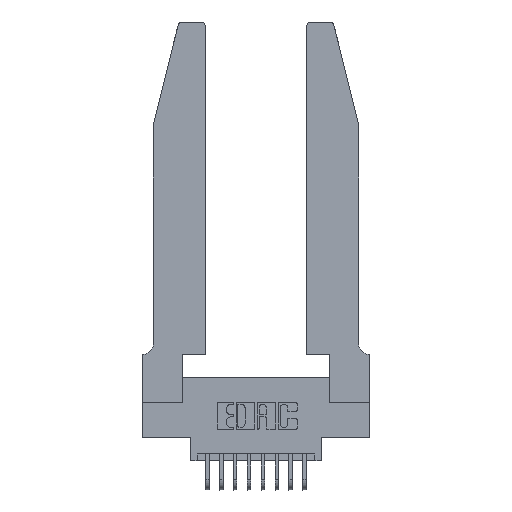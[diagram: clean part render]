
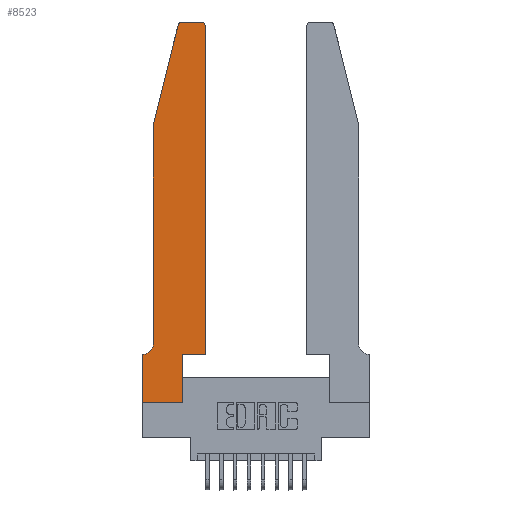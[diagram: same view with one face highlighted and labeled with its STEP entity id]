
A CAD part, top view. The second image highlights one B-rep face of the part: STEP entity #8523.
In plain terms, the highlighted planar face has unit normal (0, 0, 1).
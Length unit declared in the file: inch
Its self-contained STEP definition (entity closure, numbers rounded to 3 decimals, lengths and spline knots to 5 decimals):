
#347 = ORIENTED_EDGE ( 'NONE', *, *, #9754, .T. ) ;
#511 = CARTESIAN_POINT ( 'NONE',  ( 0.2865, 0.35, 0.37 ) ) ;
#692 = VERTEX_POINT ( 'NONE', #4070 ) ;
#704 = EDGE_CURVE ( 'NONE', #1204, #10091, #8605, .T. ) ;
#888 = ORIENTED_EDGE ( 'NONE', *, *, #15218, .T. ) ;
#1204 = VERTEX_POINT ( 'NONE', #12159 ) ;
#1240 = CARTESIAN_POINT ( 'NONE',  ( 0.0755, 2., 0.37 ) ) ;
#1251 = VECTOR ( 'NONE', #17386, 39.37008 ) ;
#1602 = CIRCLE ( 'NONE', #2156, 0.03 ) ;
#1838 = LINE ( 'NONE', #11196, #14035 ) ;
#1917 = DIRECTION ( 'NONE',  ( 1., 0., 0. ) ) ;
#1928 = CARTESIAN_POINT ( 'NONE',  ( 0., 0., 0.37 ) ) ;
#1946 = ORIENTED_EDGE ( 'NONE', *, *, #10575, .T. ) ;
#2156 = AXIS2_PLACEMENT_3D ( 'NONE', #3734, #15535, #12899 ) ;
#2363 = EDGE_CURVE ( 'NONE', #692, #7501, #1602, .T. ) ;
#2417 = CARTESIAN_POINT ( 'NONE',  ( 0.0755, 0.42, 0.37 ) ) ;
#2533 = CARTESIAN_POINT ( 'NONE',  ( 0.2865, 0.35, 0.37 ) ) ;
#2564 = AXIS2_PLACEMENT_3D ( 'NONE', #15201, #5984, #14077 ) ;
#2890 = EDGE_LOOP ( 'NONE', ( #3415, #6520, #11532, #1946, #10622, #15203, #888, #3241, #5533, #347, #11767, #4960 ) ) ;
#3067 = VECTOR ( 'NONE', #17357, 39.37008 ) ;
#3241 = ORIENTED_EDGE ( 'NONE', *, *, #15043, .T. ) ;
#3364 = CARTESIAN_POINT ( 'NONE',  ( 0.4205, 2.72, 0.37 ) ) ;
#3415 = ORIENTED_EDGE ( 'NONE', *, *, #12938, .T. ) ;
#3461 = CARTESIAN_POINT ( 'NONE',  ( 0.4205, 2.75, 0.37 ) ) ;
#3537 = CARTESIAN_POINT ( 'NONE',  ( 0., 0.35, 0.37 ) ) ;
#3642 = VECTOR ( 'NONE', #4032, 39.37008 ) ;
#3734 = CARTESIAN_POINT ( 'NONE',  ( 0.284, 2.72, 0.37 ) ) ;
#4032 = DIRECTION ( 'NONE',  ( 0., -1., 0. ) ) ;
#4070 = CARTESIAN_POINT ( 'NONE',  ( 0.284, 2.75, 0.37 ) ) ;
#4332 = FACE_OUTER_BOUND ( 'NONE', #2890, .T. ) ;
#4350 = AXIS2_PLACEMENT_3D ( 'NONE', #3364, #6073, #15453 ) ;
#4546 = LINE ( 'NONE', #6626, #3067 ) ;
#4590 = VECTOR ( 'NONE', #16129, 39.37008 ) ;
#4960 = ORIENTED_EDGE ( 'NONE', *, *, #11045, .T. ) ;
#4996 = CARTESIAN_POINT ( 'NONE',  ( 0., 0., 0.37 ) ) ;
#5533 = ORIENTED_EDGE ( 'NONE', *, *, #15753, .T. ) ;
#5984 = DIRECTION ( 'NONE',  ( 0., 0., -1. ) ) ;
#6049 = CARTESIAN_POINT ( 'NONE',  ( 0.2865, 0., 0.37 ) ) ;
#6073 = DIRECTION ( 'NONE',  ( 0., 0., 1. ) ) ;
#6252 = DIRECTION ( 'NONE',  ( 1., 0., 0. ) ) ;
#6520 = ORIENTED_EDGE ( 'NONE', *, *, #2363, .T. ) ;
#6537 = CARTESIAN_POINT ( 'NONE',  ( 0.0755, 0.35, 0.37 ) ) ;
#6626 = CARTESIAN_POINT ( 'NONE',  ( 0.4505, 0.35, 0.37 ) ) ;
#6681 = VERTEX_POINT ( 'NONE', #13858 ) ;
#6736 = CARTESIAN_POINT ( 'NONE',  ( 0.0755, 2., 0.37 ) ) ;
#7360 = VERTEX_POINT ( 'NONE', #4996 ) ;
#7501 = VERTEX_POINT ( 'NONE', #15909 ) ;
#7638 = LINE ( 'NONE', #16702, #14593 ) ;
#7845 = EDGE_CURVE ( 'NONE', #7501, #8237, #12537, .T. ) ;
#8237 = VERTEX_POINT ( 'NONE', #1240 ) ;
#8353 = LINE ( 'NONE', #1928, #9402 ) ;
#8427 = VERTEX_POINT ( 'NONE', #6049 ) ;
#8523 = ADVANCED_FACE ( 'NONE', ( #4332 ), #10274, .T. ) ;
#8605 = LINE ( 'NONE', #6537, #1251 ) ;
#8958 = VECTOR ( 'NONE', #15131, 39.37008 ) ;
#9220 = CIRCLE ( 'NONE', #2564, 0.07 ) ;
#9265 = CIRCLE ( 'NONE', #4350, 0.03 ) ;
#9402 = VECTOR ( 'NONE', #12696, 39.37008 ) ;
#9754 = EDGE_CURVE ( 'NONE', #12307, #6681, #7638, .T. ) ;
#9851 = CARTESIAN_POINT ( 'NONE',  ( 0., 0.35, 0.37 ) ) ;
#10091 = VERTEX_POINT ( 'NONE', #9851 ) ;
#10092 = VERTEX_POINT ( 'NONE', #15387 ) ;
#10274 = PLANE ( 'NONE',  #14790 ) ;
#10575 = EDGE_CURVE ( 'NONE', #8237, #10766, #15389, .T. ) ;
#10622 = ORIENTED_EDGE ( 'NONE', *, *, #12827, .T. ) ;
#10766 = VERTEX_POINT ( 'NONE', #2417 ) ;
#11045 = EDGE_CURVE ( 'NONE', #10092, #12889, #9265, .T. ) ;
#11085 = LINE ( 'NONE', #13563, #4590 ) ;
#11196 = CARTESIAN_POINT ( 'NONE',  ( 0.2605, 2.75, 0.37 ) ) ;
#11470 = LINE ( 'NONE', #511, #15471 ) ;
#11532 = ORIENTED_EDGE ( 'NONE', *, *, #7845, .T. ) ;
#11767 = ORIENTED_EDGE ( 'NONE', *, *, #16103, .T. ) ;
#12159 = CARTESIAN_POINT ( 'NONE',  ( 0.0055, 0.35, 0.37 ) ) ;
#12307 = VERTEX_POINT ( 'NONE', #2533 ) ;
#12537 = LINE ( 'NONE', #13604, #8958 ) ;
#12696 = DIRECTION ( 'NONE',  ( 0., -1., 0. ) ) ;
#12827 = EDGE_CURVE ( 'NONE', #10766, #1204, #9220, .T. ) ;
#12889 = VERTEX_POINT ( 'NONE', #3461 ) ;
#12899 = DIRECTION ( 'NONE',  ( 1., 0., 0. ) ) ;
#12938 = EDGE_CURVE ( 'NONE', #12889, #692, #1838, .T. ) ;
#13563 = CARTESIAN_POINT ( 'NONE',  ( 0., 0., 0.37 ) ) ;
#13604 = CARTESIAN_POINT ( 'NONE',  ( 0.0755, 2., 0.37 ) ) ;
#13620 = DIRECTION ( 'NONE',  ( -1., 0., 0. ) ) ;
#13858 = CARTESIAN_POINT ( 'NONE',  ( 0.4505, 0.35, 0.37 ) ) ;
#14035 = VECTOR ( 'NONE', #13620, 39.37008 ) ;
#14077 = DIRECTION ( 'NONE',  ( -1., 0., 0. ) ) ;
#14593 = VECTOR ( 'NONE', #1917, 39.37008 ) ;
#14790 = AXIS2_PLACEMENT_3D ( 'NONE', #3537, #15688, #6252 ) ;
#15043 = EDGE_CURVE ( 'NONE', #7360, #8427, #11085, .T. ) ;
#15131 = DIRECTION ( 'NONE',  ( -0.239, -0.971, 0. ) ) ;
#15201 = CARTESIAN_POINT ( 'NONE',  ( 0.0055, 0.42, 0.37 ) ) ;
#15203 = ORIENTED_EDGE ( 'NONE', *, *, #704, .T. ) ;
#15218 = EDGE_CURVE ( 'NONE', #10091, #7360, #8353, .T. ) ;
#15387 = CARTESIAN_POINT ( 'NONE',  ( 0.4505, 2.72, 0.37 ) ) ;
#15389 = LINE ( 'NONE', #6736, #3642 ) ;
#15453 = DIRECTION ( 'NONE',  ( 1., 0., 0. ) ) ;
#15471 = VECTOR ( 'NONE', #16630, 39.37008 ) ;
#15535 = DIRECTION ( 'NONE',  ( 0., 0., 1. ) ) ;
#15688 = DIRECTION ( 'NONE',  ( 0., 0., 1. ) ) ;
#15753 = EDGE_CURVE ( 'NONE', #8427, #12307, #11470, .T. ) ;
#15909 = CARTESIAN_POINT ( 'NONE',  ( 0.25487, 2.72718, 0.37 ) ) ;
#16103 = EDGE_CURVE ( 'NONE', #6681, #10092, #4546, .T. ) ;
#16129 = DIRECTION ( 'NONE',  ( 1., 0., 0. ) ) ;
#16630 = DIRECTION ( 'NONE',  ( 0., 1., 0. ) ) ;
#16702 = CARTESIAN_POINT ( 'NONE',  ( 0.4505, 0.35, 0.37 ) ) ;
#17357 = DIRECTION ( 'NONE',  ( 0., 1., 0. ) ) ;
#17386 = DIRECTION ( 'NONE',  ( -1., 0., 0. ) ) ;
